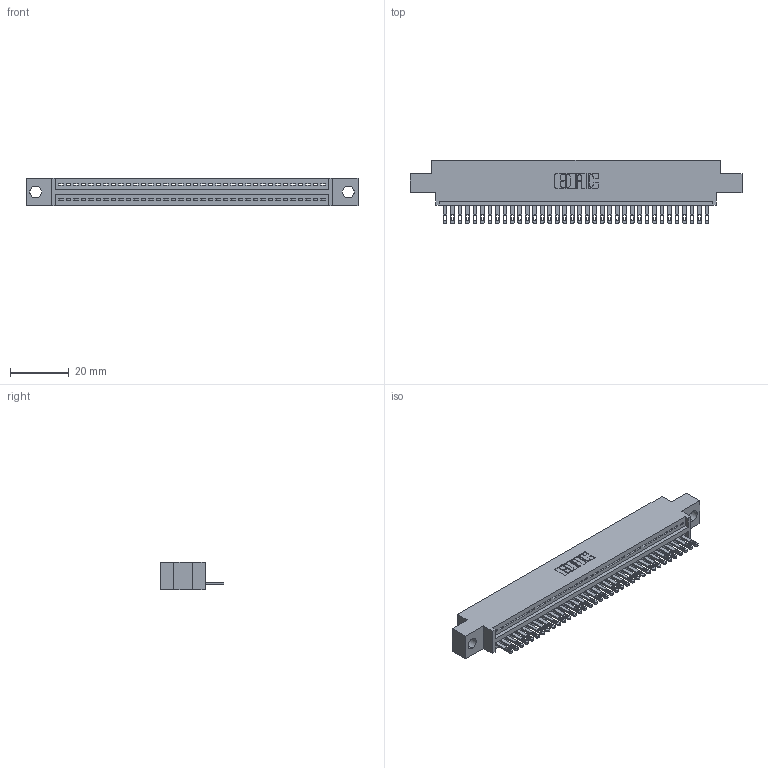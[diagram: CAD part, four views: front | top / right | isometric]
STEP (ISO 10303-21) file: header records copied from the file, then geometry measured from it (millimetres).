
FILE_DESCRIPTION (( 'STEP AP203' ), '1' );
FILE_NAME ('345-036-500-604.STEP', '2019-10-07T22:10:05', ( '' ), ( '' ), 'SwSTEP 2.0', 'SolidWorks 2016', '' );
FILE_SCHEMA (( 'CONFIG_CONTROL_DESIGN' ));
Length unit declared in the file: inch
Products named in the file (3): 345 Part_0.170 Offset - 0.156 Dia-TH; 345-036-500-604; 345-292-001_345-293-100
Assembly tree (37 placements, depth 2):
  345-036-500-604
    345 Part_0.170 Offset - 0.156 Dia-TH
    345-292-001_345-293-100  x36
Bounding box: 112.65 x 21.51 x 9.4 mm (x, y, z)
Volume: 10471.4 mm3; surface area: 13850.2 mm2
Topology: 37 solids, 37 shells, 2074 faces, 6401 edges, 4266 vertices
Faces by surface type: plane 1308, cylinder 766
Entity records: 27967 total; most frequent: CARTESIAN_POINT 4852, ORIENTED_EDGE 4822, DIRECTION 4247, EDGE_CURVE 2411, VECTOR 2131, LINE 2131, VERTEX_POINT 1606, AXIS2_PLACEMENT_3D 1058
